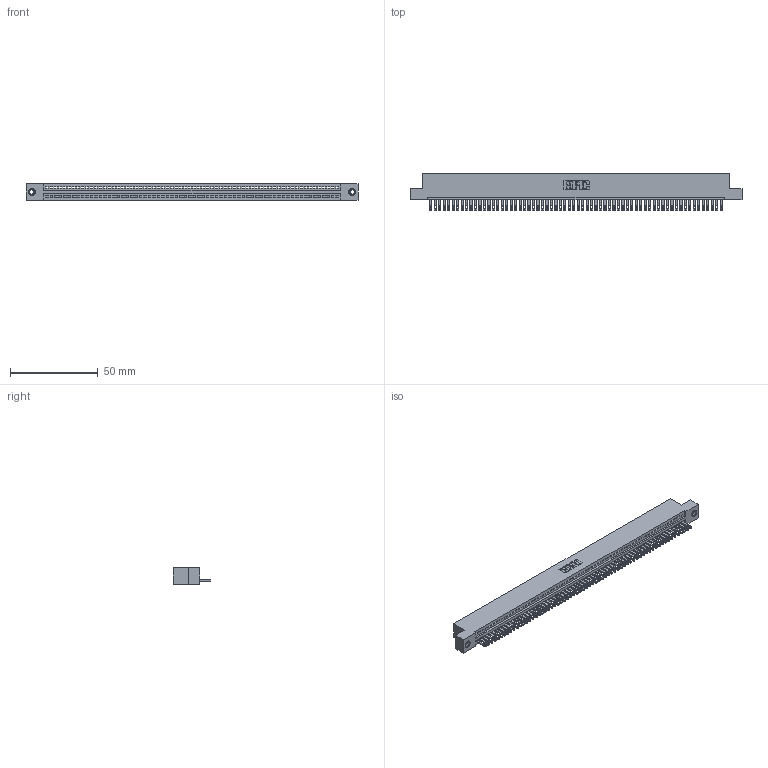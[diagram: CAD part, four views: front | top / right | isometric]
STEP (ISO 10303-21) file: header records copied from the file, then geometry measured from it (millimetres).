
FILE_DESCRIPTION (( 'STEP AP203' ), '1' );
FILE_NAME ('895-066-500-107.STEP', '2020-09-28T12:06:37', ( '' ), ( '' ), 'SwSTEP 2.0', 'SolidWorks 2020', '' );
FILE_SCHEMA (( 'CONFIG_CONTROL_DESIGN' ));
Length unit declared in the file: inch
Products named in the file (4): 895-066-500-107; 845 Part_Flush Mounting Lugs - 0.156 Dia-TI; 345-250-001_345-250-005-103; 345-292-001_345-293-100
Assembly tree (69 placements, depth 2):
  895-066-500-107
    845 Part_Flush Mounting Lugs - 0.156 Dia-TI
    345-292-001_345-293-100  x66
    345-250-001_345-250-005-103  x2
Bounding box: 188.85 x 21.51 x 9.4 mm (x, y, z)
Volume: 18161 mm3; surface area: 24641.3 mm2
Topology: 69 solids, 69 shells, 3750 faces, 11565 edges, 7702 vertices
Faces by surface type: plane 2356, cylinder 1378, cone 12, torus 4
Entity records: 47558 total; most frequent: CARTESIAN_POINT 8217, ORIENTED_EDGE 8210, DIRECTION 7171, EDGE_CURVE 4105, LINE 3685, VECTOR 3685, VERTEX_POINT 2732, AXIS2_PLACEMENT_3D 1743
